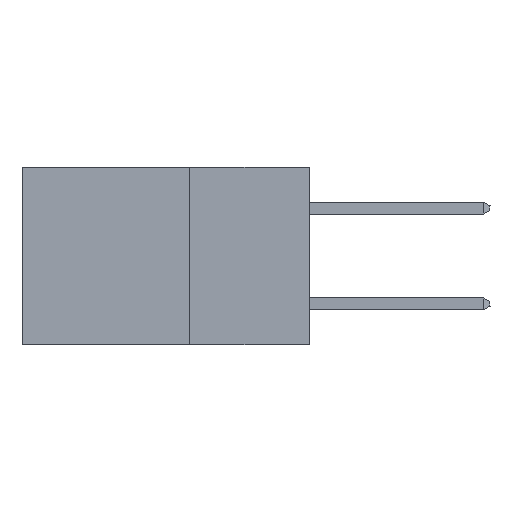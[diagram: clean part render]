
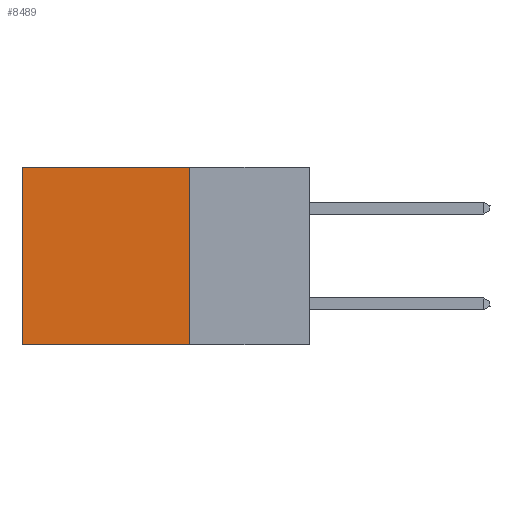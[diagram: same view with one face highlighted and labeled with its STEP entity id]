
A CAD part, left-side view. The second image highlights one B-rep face of the part: STEP entity #8489.
In plain terms, the highlighted planar face has unit normal (-1, 0, 0).
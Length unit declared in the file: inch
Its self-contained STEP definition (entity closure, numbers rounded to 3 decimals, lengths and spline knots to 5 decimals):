
#2321 = ORIENTED_EDGE ( 'NONE', *, *, #16854, .F. ) ;
#2718 = EDGE_CURVE ( 'NONE', #15003, #18463, #3690, .T. ) ;
#3090 = CARTESIAN_POINT ( 'NONE',  ( 0.2875, 0.25, 0. ) ) ;
#3342 = PLANE ( 'NONE',  #22233 ) ;
#3690 = LINE ( 'NONE', #23655, #16322 ) ;
#3797 = LINE ( 'NONE', #12829, #6649 ) ;
#6626 = FACE_OUTER_BOUND ( 'NONE', #12285, .T. ) ;
#6649 = VECTOR ( 'NONE', #7278, 39.37008 ) ;
#7170 = EDGE_CURVE ( 'NONE', #17294, #7201, #3797, .T. ) ;
#7201 = VERTEX_POINT ( 'NONE', #13308 ) ;
#7277 = CARTESIAN_POINT ( 'NONE',  ( 0.2875, 0.25, 0. ) ) ;
#7278 = DIRECTION ( 'NONE',  ( 0., 0., -1. ) ) ;
#8322 = DIRECTION ( 'NONE',  ( 0., 1., 0. ) ) ;
#8489 = ADVANCED_FACE ( 'NONE', ( #6626 ), #3342, .F. ) ;
#8886 = ORIENTED_EDGE ( 'NONE', *, *, #12801, .T. ) ;
#9168 = DIRECTION ( 'NONE',  ( 1., 0., 0. ) ) ;
#9406 = LINE ( 'NONE', #22718, #22326 ) ;
#12285 = EDGE_LOOP ( 'NONE', ( #16567, #2321, #22020, #8886 ) ) ;
#12801 = EDGE_CURVE ( 'NONE', #17294, #15003, #14215, .T. ) ;
#12829 = CARTESIAN_POINT ( 'NONE',  ( 0.2875, 0.25, 0. ) ) ;
#13308 = CARTESIAN_POINT ( 'NONE',  ( 0.2875, 0.25, -0.37 ) ) ;
#14215 = LINE ( 'NONE', #17394, #20252 ) ;
#15003 = VERTEX_POINT ( 'NONE', #22792 ) ;
#16322 = VECTOR ( 'NONE', #20035, 39.37008 ) ;
#16567 = ORIENTED_EDGE ( 'NONE', *, *, #2718, .T. ) ;
#16854 = EDGE_CURVE ( 'NONE', #7201, #18463, #9406, .T. ) ;
#17294 = VERTEX_POINT ( 'NONE', #7277 ) ;
#17394 = CARTESIAN_POINT ( 'NONE',  ( 0.2875, 0.25, 0. ) ) ;
#18463 = VERTEX_POINT ( 'NONE', #22399 ) ;
#20035 = DIRECTION ( 'NONE',  ( 0., 0., -1. ) ) ;
#20252 = VECTOR ( 'NONE', #8322, 39.37008 ) ;
#21945 = DIRECTION ( 'NONE',  ( 0., 0., -1. ) ) ;
#22020 = ORIENTED_EDGE ( 'NONE', *, *, #7170, .F. ) ;
#22233 = AXIS2_PLACEMENT_3D ( 'NONE', #3090, #9168, #21945 ) ;
#22326 = VECTOR ( 'NONE', #22485, 39.37008 ) ;
#22399 = CARTESIAN_POINT ( 'NONE',  ( 0.2875, 0.6, -0.37 ) ) ;
#22485 = DIRECTION ( 'NONE',  ( 0., 1., 0. ) ) ;
#22718 = CARTESIAN_POINT ( 'NONE',  ( 0.2875, 0.25, -0.37 ) ) ;
#22792 = CARTESIAN_POINT ( 'NONE',  ( 0.2875, 0.6, 0. ) ) ;
#23655 = CARTESIAN_POINT ( 'NONE',  ( 0.2875, 0.6, 0. ) ) ;
